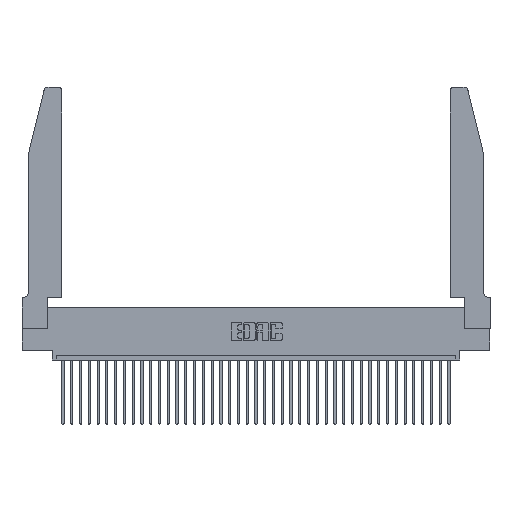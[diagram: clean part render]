
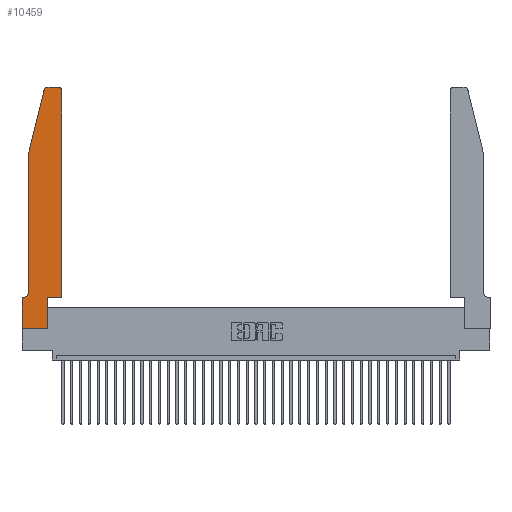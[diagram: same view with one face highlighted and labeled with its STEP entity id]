
A CAD part, top view. The second image highlights one B-rep face of the part: STEP entity #10459.
In plain terms, the highlighted planar face has unit normal (0, 0, 1).
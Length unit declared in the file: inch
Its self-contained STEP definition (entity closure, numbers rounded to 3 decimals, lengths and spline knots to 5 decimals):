
#401 = VERTEX_POINT ( 'NONE', #34278 ) ;
#1375 = LINE ( 'NONE', #15132, #2349 ) ;
#2143 = DIRECTION ( 'NONE',  ( 0., -1., 0. ) ) ;
#2158 = DIRECTION ( 'NONE',  ( 1., 0., 0. ) ) ;
#2349 = VECTOR ( 'NONE', #24254, 39.37008 ) ;
#2913 = VECTOR ( 'NONE', #26624, 39.37008 ) ;
#3528 = CARTESIAN_POINT ( 'NONE',  ( 0.4205, 2.75, 0.37 ) ) ;
#4270 = DIRECTION ( 'NONE',  ( 1., 0., 0. ) ) ;
#4624 = CARTESIAN_POINT ( 'NONE',  ( 0.0755, 2., 0.37 ) ) ;
#4660 = VECTOR ( 'NONE', #21861, 39.37008 ) ;
#4664 = VERTEX_POINT ( 'NONE', #37861 ) ;
#5346 = CARTESIAN_POINT ( 'NONE',  ( 0.284, 2.72, 0.37 ) ) ;
#5891 = CIRCLE ( 'NONE', #15053, 0.07 ) ;
#6150 = EDGE_CURVE ( 'NONE', #401, #12784, #12195, .T. ) ;
#6412 = CARTESIAN_POINT ( 'NONE',  ( 0., 0., 0.37 ) ) ;
#6710 = EDGE_CURVE ( 'NONE', #20023, #32790, #37563, .T. ) ;
#7248 = CARTESIAN_POINT ( 'NONE',  ( 0.4205, 2.72, 0.37 ) ) ;
#8283 = EDGE_CURVE ( 'NONE', #12784, #20023, #20333, .T. ) ;
#8550 = CARTESIAN_POINT ( 'NONE',  ( 0.2865, 0.35, 0.37 ) ) ;
#10090 = DIRECTION ( 'NONE',  ( 0., 1., 0. ) ) ;
#10253 = DIRECTION ( 'NONE',  ( 0., 0., 1. ) ) ;
#10459 = ADVANCED_FACE ( 'NONE', ( #18825 ), #12099, .T. ) ;
#10768 = VERTEX_POINT ( 'NONE', #27024 ) ;
#11501 = VERTEX_POINT ( 'NONE', #3528 ) ;
#11852 = LINE ( 'NONE', #21571, #23852 ) ;
#12099 = PLANE ( 'NONE',  #17585 ) ;
#12195 = LINE ( 'NONE', #23647, #2913 ) ;
#12403 = EDGE_CURVE ( 'NONE', #31930, #4664, #20689, .T. ) ;
#12784 = VERTEX_POINT ( 'NONE', #38171 ) ;
#12991 = DIRECTION ( 'NONE',  ( 1., 0., 0. ) ) ;
#13089 = EDGE_CURVE ( 'NONE', #4664, #401, #5891, .T. ) ;
#13376 = LINE ( 'NONE', #30941, #28159 ) ;
#13437 = EDGE_CURVE ( 'NONE', #19587, #31930, #32586, .T. ) ;
#13681 = ORIENTED_EDGE ( 'NONE', *, *, #19524, .T. ) ;
#13891 = CARTESIAN_POINT ( 'NONE',  ( 0.4505, 2.72, 0.37 ) ) ;
#15003 = ORIENTED_EDGE ( 'NONE', *, *, #25550, .T. ) ;
#15053 = AXIS2_PLACEMENT_3D ( 'NONE', #20334, #29125, #17410 ) ;
#15132 = CARTESIAN_POINT ( 'NONE',  ( 0.4505, 0.35, 0.37 ) ) ;
#16620 = CARTESIAN_POINT ( 'NONE',  ( 0.2865, 0., 0.37 ) ) ;
#17293 = AXIS2_PLACEMENT_3D ( 'NONE', #7248, #10253, #4270 ) ;
#17410 = DIRECTION ( 'NONE',  ( -1., 0., 0. ) ) ;
#17585 = AXIS2_PLACEMENT_3D ( 'NONE', #26690, #21833, #12991 ) ;
#18452 = CARTESIAN_POINT ( 'NONE',  ( 0.0755, 2., 0.37 ) ) ;
#18573 = DIRECTION ( 'NONE',  ( 0., -1., 0. ) ) ;
#18825 = FACE_OUTER_BOUND ( 'NONE', #21985, .T. ) ;
#18941 = CARTESIAN_POINT ( 'NONE',  ( 0.2605, 2.75, 0.37 ) ) ;
#18980 = CARTESIAN_POINT ( 'NONE',  ( 0., 0., 0.37 ) ) ;
#19364 = CIRCLE ( 'NONE', #17293, 0.03 ) ;
#19524 = EDGE_CURVE ( 'NONE', #32790, #38370, #11852, .T. ) ;
#19587 = VERTEX_POINT ( 'NONE', #21822 ) ;
#20023 = VERTEX_POINT ( 'NONE', #6412 ) ;
#20048 = ORIENTED_EDGE ( 'NONE', *, *, #8283, .T. ) ;
#20099 = VERTEX_POINT ( 'NONE', #30058 ) ;
#20333 = LINE ( 'NONE', #18980, #26336 ) ;
#20334 = CARTESIAN_POINT ( 'NONE',  ( 0.0055, 0.42, 0.37 ) ) ;
#20689 = LINE ( 'NONE', #18452, #35481 ) ;
#21548 = VERTEX_POINT ( 'NONE', #13891 ) ;
#21571 = CARTESIAN_POINT ( 'NONE',  ( 0.2865, 0.35, 0.37 ) ) ;
#21779 = DIRECTION ( 'NONE',  ( -0.239, -0.971, 0. ) ) ;
#21822 = CARTESIAN_POINT ( 'NONE',  ( 0.25487, 2.72718, 0.37 ) ) ;
#21833 = DIRECTION ( 'NONE',  ( 0., 0., 1. ) ) ;
#21861 = DIRECTION ( 'NONE',  ( -1., 0., 0. ) ) ;
#21985 = EDGE_LOOP ( 'NONE', ( #37125, #26850, #31523, #31810, #36530, #25742, #20048, #31447, #13681, #24279, #15003, #25164 ) ) ;
#23647 = CARTESIAN_POINT ( 'NONE',  ( 0.0755, 0.35, 0.37 ) ) ;
#23852 = VECTOR ( 'NONE', #10090, 39.37008 ) ;
#24254 = DIRECTION ( 'NONE',  ( 1., 0., 0. ) ) ;
#24279 = ORIENTED_EDGE ( 'NONE', *, *, #33789, .T. ) ;
#24656 = CARTESIAN_POINT ( 'NONE',  ( 0.0755, 2., 0.37 ) ) ;
#24766 = AXIS2_PLACEMENT_3D ( 'NONE', #5346, #31713, #34552 ) ;
#25164 = ORIENTED_EDGE ( 'NONE', *, *, #38083, .T. ) ;
#25385 = CIRCLE ( 'NONE', #24766, 0.03 ) ;
#25550 = EDGE_CURVE ( 'NONE', #10768, #21548, #13376, .T. ) ;
#25713 = EDGE_CURVE ( 'NONE', #20099, #19587, #25385, .T. ) ;
#25742 = ORIENTED_EDGE ( 'NONE', *, *, #6150, .T. ) ;
#26336 = VECTOR ( 'NONE', #2143, 39.37008 ) ;
#26624 = DIRECTION ( 'NONE',  ( -1., 0., 0. ) ) ;
#26690 = CARTESIAN_POINT ( 'NONE',  ( 0., 0.35, 0.37 ) ) ;
#26850 = ORIENTED_EDGE ( 'NONE', *, *, #25713, .T. ) ;
#27024 = CARTESIAN_POINT ( 'NONE',  ( 0.4505, 0.35, 0.37 ) ) ;
#27493 = VECTOR ( 'NONE', #21779, 39.37008 ) ;
#27836 = VECTOR ( 'NONE', #2158, 39.37008 ) ;
#28159 = VECTOR ( 'NONE', #33907, 39.37008 ) ;
#29125 = DIRECTION ( 'NONE',  ( 0., 0., -1. ) ) ;
#29567 = EDGE_CURVE ( 'NONE', #11501, #20099, #33341, .T. ) ;
#30058 = CARTESIAN_POINT ( 'NONE',  ( 0.284, 2.75, 0.37 ) ) ;
#30941 = CARTESIAN_POINT ( 'NONE',  ( 0.4505, 0.35, 0.37 ) ) ;
#31447 = ORIENTED_EDGE ( 'NONE', *, *, #6710, .T. ) ;
#31523 = ORIENTED_EDGE ( 'NONE', *, *, #13437, .T. ) ;
#31713 = DIRECTION ( 'NONE',  ( 0., 0., 1. ) ) ;
#31810 = ORIENTED_EDGE ( 'NONE', *, *, #12403, .T. ) ;
#31930 = VERTEX_POINT ( 'NONE', #4624 ) ;
#32586 = LINE ( 'NONE', #24656, #27493 ) ;
#32790 = VERTEX_POINT ( 'NONE', #16620 ) ;
#33341 = LINE ( 'NONE', #18941, #4660 ) ;
#33789 = EDGE_CURVE ( 'NONE', #38370, #10768, #1375, .T. ) ;
#33907 = DIRECTION ( 'NONE',  ( 0., 1., 0. ) ) ;
#34278 = CARTESIAN_POINT ( 'NONE',  ( 0.0055, 0.35, 0.37 ) ) ;
#34552 = DIRECTION ( 'NONE',  ( 1., 0., 0. ) ) ;
#35481 = VECTOR ( 'NONE', #18573, 39.37008 ) ;
#36530 = ORIENTED_EDGE ( 'NONE', *, *, #13089, .T. ) ;
#37125 = ORIENTED_EDGE ( 'NONE', *, *, #29567, .T. ) ;
#37563 = LINE ( 'NONE', #37748, #27836 ) ;
#37748 = CARTESIAN_POINT ( 'NONE',  ( 0., 0., 0.37 ) ) ;
#37861 = CARTESIAN_POINT ( 'NONE',  ( 0.0755, 0.42, 0.37 ) ) ;
#38083 = EDGE_CURVE ( 'NONE', #21548, #11501, #19364, .T. ) ;
#38171 = CARTESIAN_POINT ( 'NONE',  ( 0., 0.35, 0.37 ) ) ;
#38370 = VERTEX_POINT ( 'NONE', #8550 ) ;
